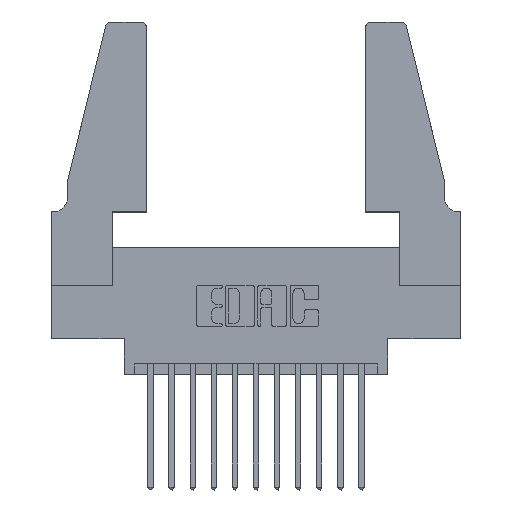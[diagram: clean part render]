
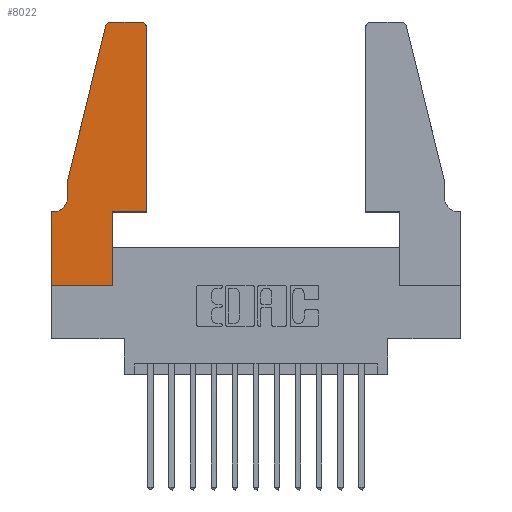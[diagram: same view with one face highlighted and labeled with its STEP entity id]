
A CAD part, top view. The second image highlights one B-rep face of the part: STEP entity #8022.
In plain terms, the highlighted planar face has unit normal (0, 0, 1).
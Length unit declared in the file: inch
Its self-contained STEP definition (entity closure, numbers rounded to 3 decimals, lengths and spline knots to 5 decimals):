
#270 = AXIS2_PLACEMENT_3D ( 'NONE', #3700, #13068, #9559 ) ;
#698 = EDGE_CURVE ( 'NONE', #4560, #7598, #5597, .T. ) ;
#756 = CARTESIAN_POINT ( 'NONE',  ( 0.2865, 0., 0.37 ) ) ;
#1379 = CARTESIAN_POINT ( 'NONE',  ( 0., 0.35, 0.37 ) ) ;
#1740 = CIRCLE ( 'NONE', #12422, 0.03 ) ;
#1750 = AXIS2_PLACEMENT_3D ( 'NONE', #9430, #10614, #3592 ) ;
#1772 = VECTOR ( 'NONE', #12264, 39.37008 ) ;
#1804 = CARTESIAN_POINT ( 'NONE',  ( 0., 0., 0.37 ) ) ;
#2032 = LINE ( 'NONE', #13170, #6570 ) ;
#2286 = VERTEX_POINT ( 'NONE', #14797 ) ;
#2607 = DIRECTION ( 'NONE',  ( 0., 0., 1. ) ) ;
#2819 = EDGE_CURVE ( 'NONE', #4273, #13153, #13443, .T. ) ;
#3418 = DIRECTION ( 'NONE',  ( 1., 0., 0. ) ) ;
#3592 = DIRECTION ( 'NONE',  ( -1., 0., 0. ) ) ;
#3700 = CARTESIAN_POINT ( 'NONE',  ( 0.4205, 1.22, 0.37 ) ) ;
#3744 = CARTESIAN_POINT ( 'NONE',  ( 0.0755, 0.35, 0.37 ) ) ;
#3867 = DIRECTION ( 'NONE',  ( -1., 0., 0. ) ) ;
#4078 = ORIENTED_EDGE ( 'NONE', *, *, #5140, .T. ) ;
#4102 = VERTEX_POINT ( 'NONE', #9554 ) ;
#4273 = VERTEX_POINT ( 'NONE', #756 ) ;
#4340 = VECTOR ( 'NONE', #8416, 39.37008 ) ;
#4431 = VERTEX_POINT ( 'NONE', #11617 ) ;
#4560 = VERTEX_POINT ( 'NONE', #11924 ) ;
#4781 = DIRECTION ( 'NONE',  ( 0., 0., 1. ) ) ;
#4923 = CARTESIAN_POINT ( 'NONE',  ( 0.284, 1.25, 0.37 ) ) ;
#5140 = EDGE_CURVE ( 'NONE', #4102, #4273, #12358, .T. ) ;
#5257 = VECTOR ( 'NONE', #14626, 39.37008 ) ;
#5278 = CARTESIAN_POINT ( 'NONE',  ( 0.4505, 1.22, 0.37 ) ) ;
#5339 = LINE ( 'NONE', #13239, #6231 ) ;
#5597 = LINE ( 'NONE', #9995, #5257 ) ;
#5828 = EDGE_CURVE ( 'NONE', #7598, #5939, #5884, .T. ) ;
#5855 = CARTESIAN_POINT ( 'NONE',  ( 0., 0.35, 0.37 ) ) ;
#5884 = CIRCLE ( 'NONE', #270, 0.03 ) ;
#5939 = VERTEX_POINT ( 'NONE', #10969 ) ;
#6231 = VECTOR ( 'NONE', #14465, 39.37008 ) ;
#6348 = CARTESIAN_POINT ( 'NONE',  ( 0.2605, 1.25, 0.37 ) ) ;
#6570 = VECTOR ( 'NONE', #13052, 39.37008 ) ;
#6621 = LINE ( 'NONE', #7441, #7533 ) ;
#6839 = CARTESIAN_POINT ( 'NONE',  ( 0.2865, 0.35, 0.37 ) ) ;
#7441 = CARTESIAN_POINT ( 'NONE',  ( 0.4505, 0.35, 0.37 ) ) ;
#7494 = EDGE_LOOP ( 'NONE', ( #12654, #7531, #12832, #15111, #14061, #13881, #8700, #4078, #10762, #8662, #9485, #12329 ) ) ;
#7531 = ORIENTED_EDGE ( 'NONE', *, *, #14026, .T. ) ;
#7533 = VECTOR ( 'NONE', #13501, 39.37008 ) ;
#7598 = VERTEX_POINT ( 'NONE', #5278 ) ;
#8022 = ADVANCED_FACE ( 'NONE', ( #9857 ), #10715, .T. ) ;
#8393 = DIRECTION ( 'NONE',  ( 1., 0., 0. ) ) ;
#8416 = DIRECTION ( 'NONE',  ( -1., 0., 0. ) ) ;
#8662 = ORIENTED_EDGE ( 'NONE', *, *, #14315, .T. ) ;
#8700 = ORIENTED_EDGE ( 'NONE', *, *, #12890, .T. ) ;
#8826 = EDGE_CURVE ( 'NONE', #5939, #12593, #14974, .T. ) ;
#9430 = CARTESIAN_POINT ( 'NONE',  ( 0.0055, 0.42, 0.37 ) ) ;
#9485 = ORIENTED_EDGE ( 'NONE', *, *, #698, .T. ) ;
#9554 = CARTESIAN_POINT ( 'NONE',  ( 0., 0., 0.37 ) ) ;
#9559 = DIRECTION ( 'NONE',  ( 1., 0., 0. ) ) ;
#9564 = CARTESIAN_POINT ( 'NONE',  ( 0.0755, 0.5, 0.37 ) ) ;
#9607 = DIRECTION ( 'NONE',  ( 0., 1., 0. ) ) ;
#9857 = FACE_OUTER_BOUND ( 'NONE', #7494, .T. ) ;
#9995 = CARTESIAN_POINT ( 'NONE',  ( 0.4505, 0.35, 0.37 ) ) ;
#10203 = VECTOR ( 'NONE', #3867, 39.37008 ) ;
#10327 = EDGE_CURVE ( 'NONE', #2286, #11550, #2032, .T. ) ;
#10389 = CARTESIAN_POINT ( 'NONE',  ( 0., 0., 0.37 ) ) ;
#10545 = CARTESIAN_POINT ( 'NONE',  ( 0.284, 1.22, 0.37 ) ) ;
#10614 = DIRECTION ( 'NONE',  ( 0., 0., -1. ) ) ;
#10715 = PLANE ( 'NONE',  #14180 ) ;
#10762 = ORIENTED_EDGE ( 'NONE', *, *, #2819, .T. ) ;
#10870 = CIRCLE ( 'NONE', #1750, 0.07 ) ;
#10969 = CARTESIAN_POINT ( 'NONE',  ( 0.4205, 1.25, 0.37 ) ) ;
#11550 = VERTEX_POINT ( 'NONE', #9564 ) ;
#11617 = CARTESIAN_POINT ( 'NONE',  ( 0.0755, 0.42, 0.37 ) ) ;
#11924 = CARTESIAN_POINT ( 'NONE',  ( 0.4505, 0.35, 0.37 ) ) ;
#12091 = EDGE_CURVE ( 'NONE', #13022, #14113, #14401, .T. ) ;
#12264 = DIRECTION ( 'NONE',  ( 0., -1., 0. ) ) ;
#12329 = ORIENTED_EDGE ( 'NONE', *, *, #5828, .T. ) ;
#12358 = LINE ( 'NONE', #10389, #13968 ) ;
#12422 = AXIS2_PLACEMENT_3D ( 'NONE', #10545, #2607, #8393 ) ;
#12593 = VERTEX_POINT ( 'NONE', #4923 ) ;
#12654 = ORIENTED_EDGE ( 'NONE', *, *, #8826, .T. ) ;
#12832 = ORIENTED_EDGE ( 'NONE', *, *, #10327, .T. ) ;
#12890 = EDGE_CURVE ( 'NONE', #14113, #4102, #13088, .T. ) ;
#13022 = VERTEX_POINT ( 'NONE', #13627 ) ;
#13052 = DIRECTION ( 'NONE',  ( -0.239, -0.971, 0. ) ) ;
#13068 = DIRECTION ( 'NONE',  ( 0., 0., 1. ) ) ;
#13088 = LINE ( 'NONE', #1804, #1772 ) ;
#13153 = VERTEX_POINT ( 'NONE', #6839 ) ;
#13170 = CARTESIAN_POINT ( 'NONE',  ( 0.0755, 0.5, 0.37 ) ) ;
#13239 = CARTESIAN_POINT ( 'NONE',  ( 0.0755, 0.5, 0.37 ) ) ;
#13348 = EDGE_CURVE ( 'NONE', #4431, #13022, #10870, .T. ) ;
#13443 = LINE ( 'NONE', #14850, #14551 ) ;
#13501 = DIRECTION ( 'NONE',  ( 1., 0., 0. ) ) ;
#13627 = CARTESIAN_POINT ( 'NONE',  ( 0.0055, 0.35, 0.37 ) ) ;
#13881 = ORIENTED_EDGE ( 'NONE', *, *, #12091, .T. ) ;
#13968 = VECTOR ( 'NONE', #3418, 39.37008 ) ;
#14026 = EDGE_CURVE ( 'NONE', #12593, #2286, #1740, .T. ) ;
#14043 = DIRECTION ( 'NONE',  ( 1., 0., 0. ) ) ;
#14061 = ORIENTED_EDGE ( 'NONE', *, *, #13348, .T. ) ;
#14113 = VERTEX_POINT ( 'NONE', #5855 ) ;
#14180 = AXIS2_PLACEMENT_3D ( 'NONE', #1379, #4781, #14043 ) ;
#14315 = EDGE_CURVE ( 'NONE', #13153, #4560, #6621, .T. ) ;
#14401 = LINE ( 'NONE', #3744, #4340 ) ;
#14465 = DIRECTION ( 'NONE',  ( 0., -1., 0. ) ) ;
#14551 = VECTOR ( 'NONE', #9607, 39.37008 ) ;
#14626 = DIRECTION ( 'NONE',  ( 0., 1., 0. ) ) ;
#14797 = CARTESIAN_POINT ( 'NONE',  ( 0.25487, 1.22718, 0.37 ) ) ;
#14850 = CARTESIAN_POINT ( 'NONE',  ( 0.2865, 0.35, 0.37 ) ) ;
#14924 = EDGE_CURVE ( 'NONE', #11550, #4431, #5339, .T. ) ;
#14974 = LINE ( 'NONE', #6348, #10203 ) ;
#15111 = ORIENTED_EDGE ( 'NONE', *, *, #14924, .T. ) ;
